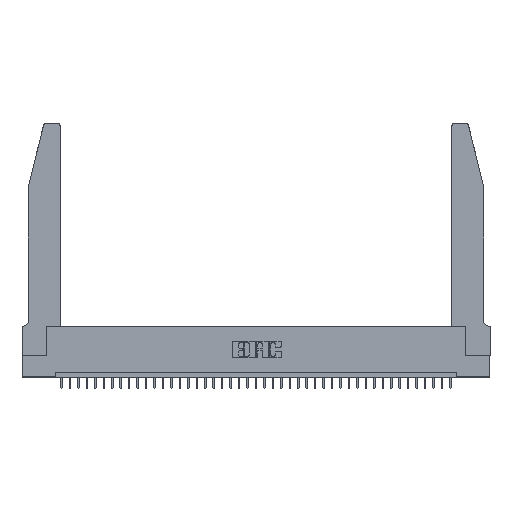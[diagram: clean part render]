
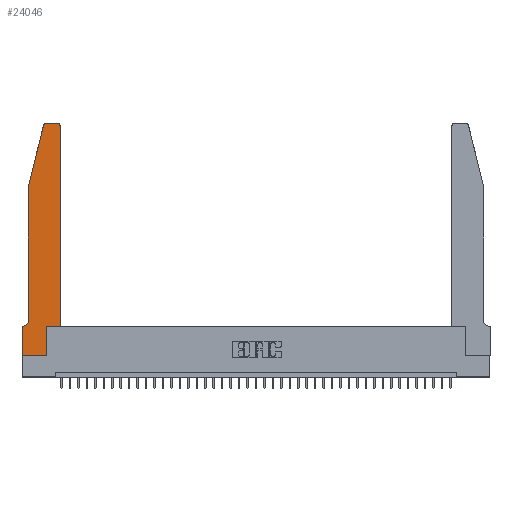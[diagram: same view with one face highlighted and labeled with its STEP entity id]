
A CAD part, top view. The second image highlights one B-rep face of the part: STEP entity #24046.
In plain terms, the highlighted planar face has unit normal (0, 0, 1).
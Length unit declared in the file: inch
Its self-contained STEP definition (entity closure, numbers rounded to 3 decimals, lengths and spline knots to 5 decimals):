
#142 = LINE ( 'NONE', #3355, #29445 ) ;
#726 = CARTESIAN_POINT ( 'NONE',  ( 0.25487, 2.72718, 0.37 ) ) ;
#1227 = CARTESIAN_POINT ( 'NONE',  ( 0., 0., 0.37 ) ) ;
#1299 = LINE ( 'NONE', #32333, #2559 ) ;
#2166 = CARTESIAN_POINT ( 'NONE',  ( 0.4205, 2.72, 0.37 ) ) ;
#2559 = VECTOR ( 'NONE', #26123, 39.37008 ) ;
#2722 = CARTESIAN_POINT ( 'NONE',  ( 0.0755, 2., 0.37 ) ) ;
#3355 = CARTESIAN_POINT ( 'NONE',  ( 0., 0., 0.37 ) ) ;
#3810 = CARTESIAN_POINT ( 'NONE',  ( 0.284, 2.72, 0.37 ) ) ;
#3928 = ORIENTED_EDGE ( 'NONE', *, *, #5299, .T. ) ;
#4981 = ORIENTED_EDGE ( 'NONE', *, *, #7797, .T. ) ;
#5299 = EDGE_CURVE ( 'NONE', #8793, #39403, #18408, .T. ) ;
#5305 = PLANE ( 'NONE',  #31389 ) ;
#5561 = DIRECTION ( 'NONE',  ( 0., -1., 0. ) ) ;
#5621 = LINE ( 'NONE', #36026, #32201 ) ;
#6312 = DIRECTION ( 'NONE',  ( -1., 0., 0. ) ) ;
#6763 = VECTOR ( 'NONE', #9050, 39.37008 ) ;
#7021 = VERTEX_POINT ( 'NONE', #34832 ) ;
#7797 = EDGE_CURVE ( 'NONE', #34883, #38277, #14395, .T. ) ;
#8221 = CARTESIAN_POINT ( 'NONE',  ( 0.4505, 2.72, 0.37 ) ) ;
#8330 = EDGE_CURVE ( 'NONE', #9193, #21007, #1299, .T. ) ;
#8633 = DIRECTION ( 'NONE',  ( 1., 0., 0. ) ) ;
#8657 = ORIENTED_EDGE ( 'NONE', *, *, #28301, .T. ) ;
#8711 = AXIS2_PLACEMENT_3D ( 'NONE', #3810, #9446, #21633 ) ;
#8793 = VERTEX_POINT ( 'NONE', #24988 ) ;
#9033 = EDGE_CURVE ( 'NONE', #7021, #34883, #142, .T. ) ;
#9050 = DIRECTION ( 'NONE',  ( 0., 1., 0. ) ) ;
#9193 = VERTEX_POINT ( 'NONE', #726 ) ;
#9446 = DIRECTION ( 'NONE',  ( 0., 0., 1. ) ) ;
#9771 = VERTEX_POINT ( 'NONE', #16523 ) ;
#10041 = ORIENTED_EDGE ( 'NONE', *, *, #32931, .T. ) ;
#10691 = ORIENTED_EDGE ( 'NONE', *, *, #30852, .T. ) ;
#10991 = DIRECTION ( 'NONE',  ( 0., 0., 1. ) ) ;
#12321 = CARTESIAN_POINT ( 'NONE',  ( 0.0755, 0.35, 0.37 ) ) ;
#13100 = VECTOR ( 'NONE', #6312, 39.37008 ) ;
#13436 = EDGE_CURVE ( 'NONE', #38277, #29615, #23314, .T. ) ;
#13942 = CARTESIAN_POINT ( 'NONE',  ( 0.2865, 0.35, 0.37 ) ) ;
#14345 = ORIENTED_EDGE ( 'NONE', *, *, #30176, .T. ) ;
#14395 = LINE ( 'NONE', #20383, #26173 ) ;
#14526 = CARTESIAN_POINT ( 'NONE',  ( 0., 0.35, 0.37 ) ) ;
#14572 = VERTEX_POINT ( 'NONE', #31988 ) ;
#15012 = DIRECTION ( 'NONE',  ( 1., 0., 0. ) ) ;
#15236 = AXIS2_PLACEMENT_3D ( 'NONE', #18860, #21861, #24850 ) ;
#16220 = VECTOR ( 'NONE', #28917, 39.37008 ) ;
#16523 = CARTESIAN_POINT ( 'NONE',  ( 0.4205, 2.75, 0.37 ) ) ;
#16880 = EDGE_LOOP ( 'NONE', ( #10041, #25218, #32380, #8657, #3928, #14345, #30720, #4981, #37465, #17928, #10691, #30857 ) ) ;
#17928 = ORIENTED_EDGE ( 'NONE', *, *, #36959, .T. ) ;
#18408 = CIRCLE ( 'NONE', #15236, 0.07 ) ;
#18438 = LINE ( 'NONE', #33832, #6763 ) ;
#18860 = CARTESIAN_POINT ( 'NONE',  ( 0.0055, 0.42, 0.37 ) ) ;
#19327 = CARTESIAN_POINT ( 'NONE',  ( 0.2605, 2.75, 0.37 ) ) ;
#19519 = CARTESIAN_POINT ( 'NONE',  ( 0.0055, 0.35, 0.37 ) ) ;
#20383 = CARTESIAN_POINT ( 'NONE',  ( 0., 0., 0.37 ) ) ;
#20386 = EDGE_CURVE ( 'NONE', #32222, #9771, #24131, .T. ) ;
#20992 = DIRECTION ( 'NONE',  ( 0., -1., 0. ) ) ;
#21007 = VERTEX_POINT ( 'NONE', #2722 ) ;
#21080 = CARTESIAN_POINT ( 'NONE',  ( 0.2865, 0., 0.37 ) ) ;
#21633 = DIRECTION ( 'NONE',  ( 1., 0., 0. ) ) ;
#21861 = DIRECTION ( 'NONE',  ( 0., 0., -1. ) ) ;
#23296 = DIRECTION ( 'NONE',  ( 1., 0., 0. ) ) ;
#23314 = LINE ( 'NONE', #13942, #16220 ) ;
#23549 = CARTESIAN_POINT ( 'NONE',  ( 0.0755, 2., 0.37 ) ) ;
#24046 = ADVANCED_FACE ( 'NONE', ( #35317 ), #5305, .T. ) ;
#24131 = CIRCLE ( 'NONE', #29870, 0.03 ) ;
#24850 = DIRECTION ( 'NONE',  ( -1., 0., 0. ) ) ;
#24988 = CARTESIAN_POINT ( 'NONE',  ( 0.0755, 0.42, 0.37 ) ) ;
#25218 = ORIENTED_EDGE ( 'NONE', *, *, #30819, .T. ) ;
#25316 = LINE ( 'NONE', #19327, #33916 ) ;
#25576 = VERTEX_POINT ( 'NONE', #34694 ) ;
#25919 = CIRCLE ( 'NONE', #8711, 0.03 ) ;
#26123 = DIRECTION ( 'NONE',  ( -0.239, -0.971, 0. ) ) ;
#26173 = VECTOR ( 'NONE', #35396, 39.37008 ) ;
#27684 = LINE ( 'NONE', #12321, #13100 ) ;
#28301 = EDGE_CURVE ( 'NONE', #21007, #8793, #29543, .T. ) ;
#28917 = DIRECTION ( 'NONE',  ( 0., 1., 0. ) ) ;
#29445 = VECTOR ( 'NONE', #20992, 39.37008 ) ;
#29543 = LINE ( 'NONE', #23549, #36640 ) ;
#29615 = VERTEX_POINT ( 'NONE', #38348 ) ;
#29693 = DIRECTION ( 'NONE',  ( 0., 0., 1. ) ) ;
#29870 = AXIS2_PLACEMENT_3D ( 'NONE', #2166, #10991, #15012 ) ;
#30176 = EDGE_CURVE ( 'NONE', #39403, #7021, #27684, .T. ) ;
#30720 = ORIENTED_EDGE ( 'NONE', *, *, #9033, .T. ) ;
#30819 = EDGE_CURVE ( 'NONE', #14572, #9193, #25919, .T. ) ;
#30852 = EDGE_CURVE ( 'NONE', #25576, #32222, #18438, .T. ) ;
#30857 = ORIENTED_EDGE ( 'NONE', *, *, #20386, .T. ) ;
#31389 = AXIS2_PLACEMENT_3D ( 'NONE', #14526, #29693, #23296 ) ;
#31988 = CARTESIAN_POINT ( 'NONE',  ( 0.284, 2.75, 0.37 ) ) ;
#32201 = VECTOR ( 'NONE', #8633, 39.37008 ) ;
#32222 = VERTEX_POINT ( 'NONE', #8221 ) ;
#32333 = CARTESIAN_POINT ( 'NONE',  ( 0.0755, 2., 0.37 ) ) ;
#32380 = ORIENTED_EDGE ( 'NONE', *, *, #8330, .T. ) ;
#32931 = EDGE_CURVE ( 'NONE', #9771, #14572, #25316, .T. ) ;
#33832 = CARTESIAN_POINT ( 'NONE',  ( 0.4505, 0.35, 0.37 ) ) ;
#33916 = VECTOR ( 'NONE', #34741, 39.37008 ) ;
#34694 = CARTESIAN_POINT ( 'NONE',  ( 0.4505, 0.35, 0.37 ) ) ;
#34741 = DIRECTION ( 'NONE',  ( -1., 0., 0. ) ) ;
#34832 = CARTESIAN_POINT ( 'NONE',  ( 0., 0.35, 0.37 ) ) ;
#34883 = VERTEX_POINT ( 'NONE', #1227 ) ;
#35317 = FACE_OUTER_BOUND ( 'NONE', #16880, .T. ) ;
#35396 = DIRECTION ( 'NONE',  ( 1., 0., 0. ) ) ;
#36026 = CARTESIAN_POINT ( 'NONE',  ( 0.4505, 0.35, 0.37 ) ) ;
#36640 = VECTOR ( 'NONE', #5561, 39.37008 ) ;
#36959 = EDGE_CURVE ( 'NONE', #29615, #25576, #5621, .T. ) ;
#37465 = ORIENTED_EDGE ( 'NONE', *, *, #13436, .T. ) ;
#38277 = VERTEX_POINT ( 'NONE', #21080 ) ;
#38348 = CARTESIAN_POINT ( 'NONE',  ( 0.2865, 0.35, 0.37 ) ) ;
#39403 = VERTEX_POINT ( 'NONE', #19519 ) ;
